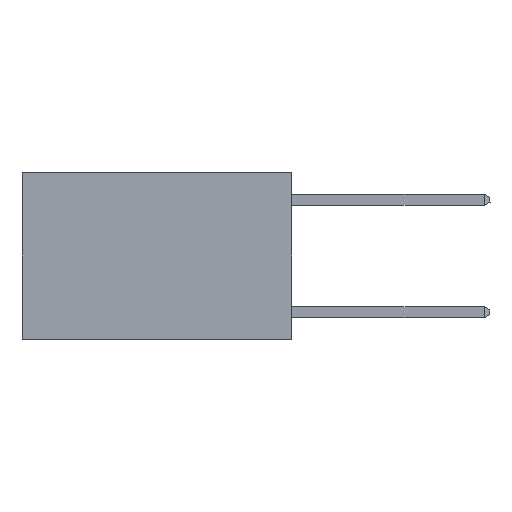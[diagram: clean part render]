
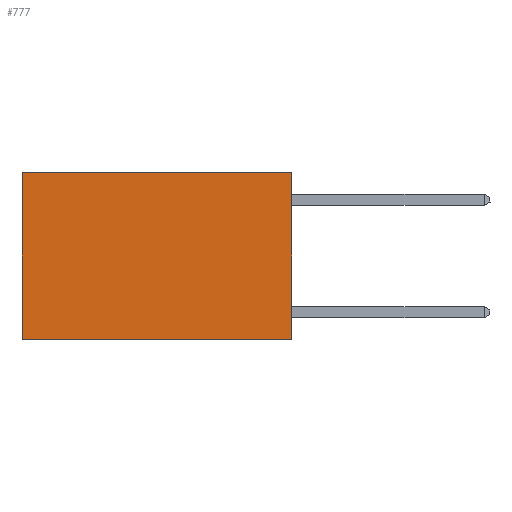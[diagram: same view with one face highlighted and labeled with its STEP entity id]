
A CAD part, left-side view. The second image highlights one B-rep face of the part: STEP entity #777.
In plain terms, the highlighted planar face has unit normal (-1, 0, 0).
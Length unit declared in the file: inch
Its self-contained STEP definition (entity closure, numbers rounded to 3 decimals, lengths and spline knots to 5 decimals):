
#591 = DIRECTION ( 'NONE',  ( 0., 0., -1. ) ) ;
#777 = ADVANCED_FACE ( 'NONE', ( #5683 ), #6080, .F. ) ;
#1701 = VECTOR ( 'NONE', #1964, 39.37008 ) ;
#1964 = DIRECTION ( 'NONE',  ( 0., 0., -1. ) ) ;
#1971 = LINE ( 'NONE', #10314, #9944 ) ;
#2026 = LINE ( 'NONE', #7086, #7897 ) ;
#2178 = LINE ( 'NONE', #6492, #6188 ) ;
#2335 = CARTESIAN_POINT ( 'NONE',  ( 0.2625, 0., 0. ) ) ;
#3411 = AXIS2_PLACEMENT_3D ( 'NONE', #6494, #6078, #6011 ) ;
#4116 = CARTESIAN_POINT ( 'NONE',  ( 0.2625, 0.6, -0.37 ) ) ;
#4389 = CARTESIAN_POINT ( 'NONE',  ( 0.2625, 0.6, 0. ) ) ;
#4546 = VERTEX_POINT ( 'NONE', #5215 ) ;
#5215 = CARTESIAN_POINT ( 'NONE',  ( 0.2625, 0., -0.37 ) ) ;
#5437 = VERTEX_POINT ( 'NONE', #2335 ) ;
#5683 = FACE_OUTER_BOUND ( 'NONE', #10023, .T. ) ;
#6000 = LINE ( 'NONE', #4389, #1701 ) ;
#6011 = DIRECTION ( 'NONE',  ( 0., 0., -1. ) ) ;
#6078 = DIRECTION ( 'NONE',  ( 1., 0., 0. ) ) ;
#6080 = PLANE ( 'NONE',  #3411 ) ;
#6188 = VECTOR ( 'NONE', #8042, 39.37008 ) ;
#6326 = EDGE_CURVE ( 'NONE', #5437, #6872, #2178, .T. ) ;
#6492 = CARTESIAN_POINT ( 'NONE',  ( 0.2625, 0., 0. ) ) ;
#6494 = CARTESIAN_POINT ( 'NONE',  ( 0.2625, 0., 0. ) ) ;
#6872 = VERTEX_POINT ( 'NONE', #7816 ) ;
#7085 = ORIENTED_EDGE ( 'NONE', *, *, #9797, .T. ) ;
#7086 = CARTESIAN_POINT ( 'NONE',  ( 0.2625, 0., -0.37 ) ) ;
#7104 = ORIENTED_EDGE ( 'NONE', *, *, #7609, .F. ) ;
#7342 = ORIENTED_EDGE ( 'NONE', *, *, #10300, .F. ) ;
#7477 = ORIENTED_EDGE ( 'NONE', *, *, #6326, .T. ) ;
#7609 = EDGE_CURVE ( 'NONE', #4546, #9442, #2026, .T. ) ;
#7816 = CARTESIAN_POINT ( 'NONE',  ( 0.2625, 0.6, 0. ) ) ;
#7897 = VECTOR ( 'NONE', #8663, 39.37008 ) ;
#8042 = DIRECTION ( 'NONE',  ( 0., 1., 0. ) ) ;
#8663 = DIRECTION ( 'NONE',  ( 0., 1., 0. ) ) ;
#9442 = VERTEX_POINT ( 'NONE', #4116 ) ;
#9797 = EDGE_CURVE ( 'NONE', #6872, #9442, #6000, .T. ) ;
#9944 = VECTOR ( 'NONE', #591, 39.37008 ) ;
#10023 = EDGE_LOOP ( 'NONE', ( #7085, #7104, #7342, #7477 ) ) ;
#10300 = EDGE_CURVE ( 'NONE', #5437, #4546, #1971, .T. ) ;
#10314 = CARTESIAN_POINT ( 'NONE',  ( 0.2625, 0., 0. ) ) ;
